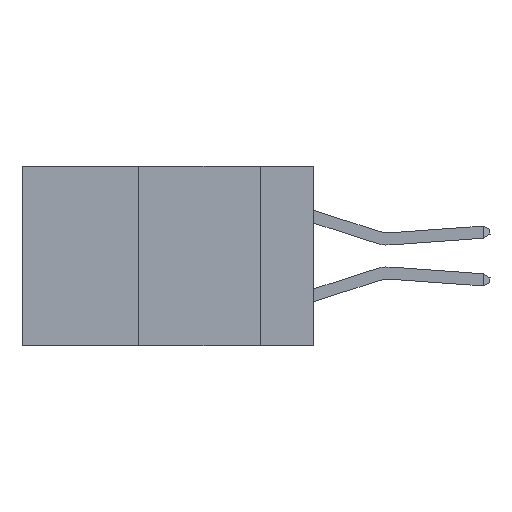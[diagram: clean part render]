
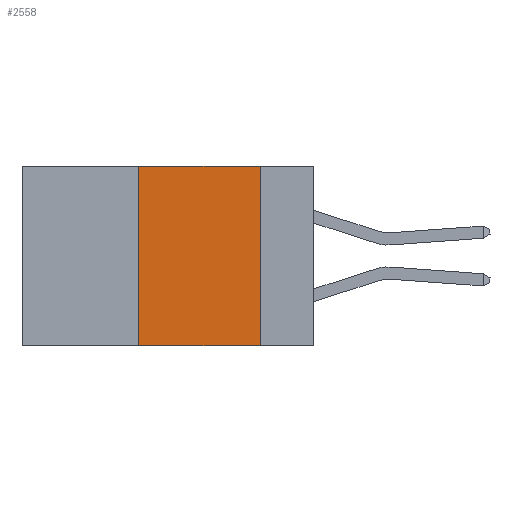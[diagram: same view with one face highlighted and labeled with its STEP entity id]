
A CAD part, left-side view. The second image highlights one B-rep face of the part: STEP entity #2558.
In plain terms, the highlighted planar face has unit normal (-1, 0, 0).
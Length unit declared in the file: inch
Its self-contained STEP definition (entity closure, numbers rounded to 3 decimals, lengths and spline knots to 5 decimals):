
#65 = LINE ( 'NONE', #10354, #9528 ) ;
#743 = CARTESIAN_POINT ( 'NONE',  ( 0., 0.36, 0. ) ) ;
#1356 = VERTEX_POINT ( 'NONE', #2889 ) ;
#1660 = VECTOR ( 'NONE', #4419, 39.37008 ) ;
#1670 = DIRECTION ( 'NONE',  ( 1., 0., 0. ) ) ;
#2178 = VERTEX_POINT ( 'NONE', #9319 ) ;
#2301 = ORIENTED_EDGE ( 'NONE', *, *, #2603, .F. ) ;
#2434 = CARTESIAN_POINT ( 'NONE',  ( 0., 0.11, 0. ) ) ;
#2512 = LINE ( 'NONE', #743, #1660 ) ;
#2558 = ADVANCED_FACE ( 'NONE', ( #8836 ), #7969, .F. ) ;
#2603 = EDGE_CURVE ( 'NONE', #1356, #3977, #2512, .T. ) ;
#2623 = CARTESIAN_POINT ( 'NONE',  ( 0., 0.6, 0. ) ) ;
#2889 = CARTESIAN_POINT ( 'NONE',  ( 0., 0.36, -0.37 ) ) ;
#3536 = EDGE_CURVE ( 'NONE', #2178, #5642, #8423, .T. ) ;
#3977 = VERTEX_POINT ( 'NONE', #4417 ) ;
#4068 = ORIENTED_EDGE ( 'NONE', *, *, #5231, .F. ) ;
#4417 = CARTESIAN_POINT ( 'NONE',  ( 0., 0.36, 0. ) ) ;
#4419 = DIRECTION ( 'NONE',  ( 0., 0., 1. ) ) ;
#5231 = EDGE_CURVE ( 'NONE', #3977, #2178, #65, .T. ) ;
#5642 = VERTEX_POINT ( 'NONE', #9080 ) ;
#5764 = ORIENTED_EDGE ( 'NONE', *, *, #11079, .T. ) ;
#5851 = DIRECTION ( 'NONE',  ( 0., -1., 0. ) ) ;
#6068 = EDGE_LOOP ( 'NONE', ( #11134, #4068, #2301, #5764 ) ) ;
#6151 = CARTESIAN_POINT ( 'NONE',  ( 0., 0.6, -0.37 ) ) ;
#7008 = VECTOR ( 'NONE', #8759, 39.37008 ) ;
#7053 = DIRECTION ( 'NONE',  ( 0., -1., 0. ) ) ;
#7449 = AXIS2_PLACEMENT_3D ( 'NONE', #2623, #1670, #7898 ) ;
#7898 = DIRECTION ( 'NONE',  ( 0., 0., -1. ) ) ;
#7969 = PLANE ( 'NONE',  #7449 ) ;
#8423 = LINE ( 'NONE', #2434, #7008 ) ;
#8614 = LINE ( 'NONE', #6151, #9922 ) ;
#8759 = DIRECTION ( 'NONE',  ( 0., 0., -1. ) ) ;
#8836 = FACE_OUTER_BOUND ( 'NONE', #6068, .T. ) ;
#9080 = CARTESIAN_POINT ( 'NONE',  ( 0., 0.11, -0.37 ) ) ;
#9319 = CARTESIAN_POINT ( 'NONE',  ( 0., 0.11, 0. ) ) ;
#9528 = VECTOR ( 'NONE', #5851, 39.37008 ) ;
#9922 = VECTOR ( 'NONE', #7053, 39.37008 ) ;
#10354 = CARTESIAN_POINT ( 'NONE',  ( 0., 0.6, 0. ) ) ;
#11079 = EDGE_CURVE ( 'NONE', #1356, #5642, #8614, .T. ) ;
#11134 = ORIENTED_EDGE ( 'NONE', *, *, #3536, .F. ) ;
